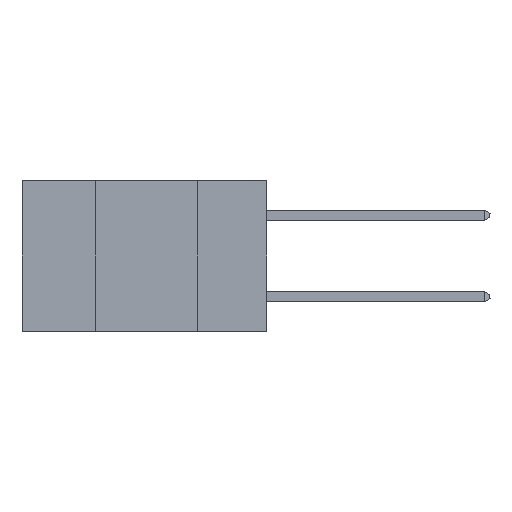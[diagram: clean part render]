
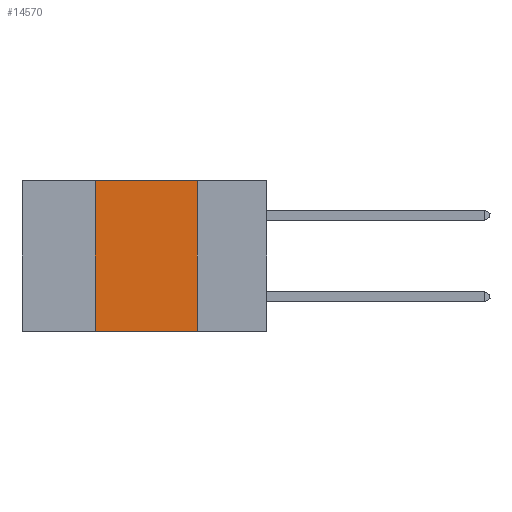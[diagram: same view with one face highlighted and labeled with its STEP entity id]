
A CAD part, left-side view. The second image highlights one B-rep face of the part: STEP entity #14570.
In plain terms, the highlighted planar face has unit normal (-1, 0, 0).
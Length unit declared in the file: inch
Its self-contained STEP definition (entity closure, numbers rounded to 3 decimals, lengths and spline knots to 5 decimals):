
#972 = CARTESIAN_POINT ( 'NONE',  ( 0., 0.42, -0.37 ) ) ;
#1078 = EDGE_LOOP ( 'NONE', ( #1497, #1486, #10810, #7214 ) ) ;
#1325 = CARTESIAN_POINT ( 'NONE',  ( 0., 0.6, 0. ) ) ;
#1486 = ORIENTED_EDGE ( 'NONE', *, *, #4069, .F. ) ;
#1497 = ORIENTED_EDGE ( 'NONE', *, *, #8190, .F. ) ;
#1543 = DIRECTION ( 'NONE',  ( 0., 0., -1. ) ) ;
#1633 = VERTEX_POINT ( 'NONE', #972 ) ;
#1947 = AXIS2_PLACEMENT_3D ( 'NONE', #1325, #14544, #4707 ) ;
#2973 = LINE ( 'NONE', #9465, #11264 ) ;
#3852 = DIRECTION ( 'NONE',  ( 0., -1., 0. ) ) ;
#4069 = EDGE_CURVE ( 'NONE', #13498, #10733, #14402, .T. ) ;
#4174 = CARTESIAN_POINT ( 'NONE',  ( 0., 0.42, 0. ) ) ;
#4313 = LINE ( 'NONE', #4174, #21175 ) ;
#4361 = LINE ( 'NONE', #13139, #20708 ) ;
#4707 = DIRECTION ( 'NONE',  ( 0., 0., -1. ) ) ;
#5841 = DIRECTION ( 'NONE',  ( 0., 0., 1. ) ) ;
#6351 = CARTESIAN_POINT ( 'NONE',  ( 0., 0.42, 0. ) ) ;
#7214 = ORIENTED_EDGE ( 'NONE', *, *, #15675, .T. ) ;
#8190 = EDGE_CURVE ( 'NONE', #10733, #16089, #4361, .T. ) ;
#9465 = CARTESIAN_POINT ( 'NONE',  ( 0., 0.6, -0.37 ) ) ;
#10073 = VECTOR ( 'NONE', #3852, 39.37008 ) ;
#10733 = VERTEX_POINT ( 'NONE', #10836 ) ;
#10810 = ORIENTED_EDGE ( 'NONE', *, *, #14996, .F. ) ;
#10836 = CARTESIAN_POINT ( 'NONE',  ( 0., 0.17, 0. ) ) ;
#11264 = VECTOR ( 'NONE', #20795, 39.37008 ) ;
#12008 = CARTESIAN_POINT ( 'NONE',  ( 0., 0.17, -0.37 ) ) ;
#12921 = PLANE ( 'NONE',  #1947 ) ;
#13139 = CARTESIAN_POINT ( 'NONE',  ( 0., 0.17, 0. ) ) ;
#13498 = VERTEX_POINT ( 'NONE', #6351 ) ;
#14402 = LINE ( 'NONE', #20147, #10073 ) ;
#14544 = DIRECTION ( 'NONE',  ( 1., 0., 0. ) ) ;
#14570 = ADVANCED_FACE ( 'NONE', ( #16896 ), #12921, .F. ) ;
#14996 = EDGE_CURVE ( 'NONE', #1633, #13498, #4313, .T. ) ;
#15675 = EDGE_CURVE ( 'NONE', #1633, #16089, #2973, .T. ) ;
#16089 = VERTEX_POINT ( 'NONE', #12008 ) ;
#16896 = FACE_OUTER_BOUND ( 'NONE', #1078, .T. ) ;
#20147 = CARTESIAN_POINT ( 'NONE',  ( 0., 0.6, 0. ) ) ;
#20708 = VECTOR ( 'NONE', #1543, 39.37008 ) ;
#20795 = DIRECTION ( 'NONE',  ( 0., -1., 0. ) ) ;
#21175 = VECTOR ( 'NONE', #5841, 39.37008 ) ;
